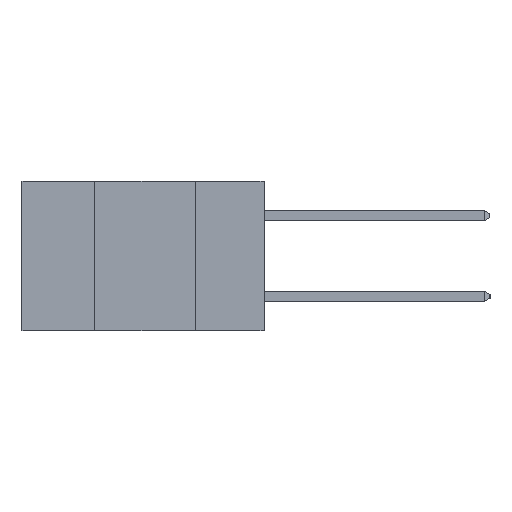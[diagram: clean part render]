
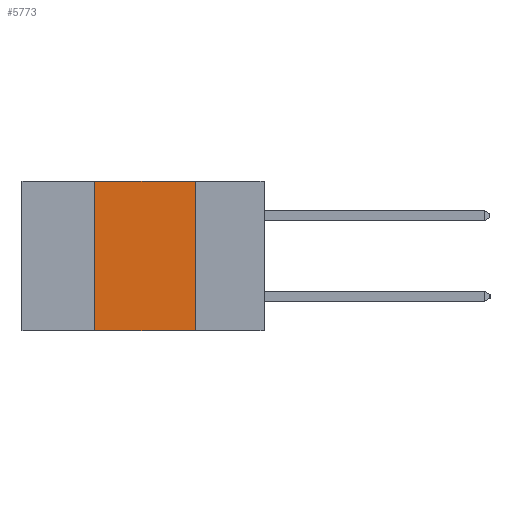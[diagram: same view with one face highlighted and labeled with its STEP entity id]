
A CAD part, left-side view. The second image highlights one B-rep face of the part: STEP entity #5773.
In plain terms, the highlighted planar face has unit normal (-1, 0, 0).
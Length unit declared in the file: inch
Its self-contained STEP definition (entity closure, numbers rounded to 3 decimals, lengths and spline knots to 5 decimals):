
#459 = LINE ( 'NONE', #12350, #6784 ) ;
#1414 = DIRECTION ( 'NONE',  ( 0., -1., 0. ) ) ;
#1646 = ORIENTED_EDGE ( 'NONE', *, *, #6915, .F. ) ;
#1975 = DIRECTION ( 'NONE',  ( 0., 0., -1. ) ) ;
#2228 = DIRECTION ( 'NONE',  ( 0., -1., 0. ) ) ;
#2509 = ORIENTED_EDGE ( 'NONE', *, *, #5936, .T. ) ;
#3166 = PLANE ( 'NONE',  #3678 ) ;
#3678 = AXIS2_PLACEMENT_3D ( 'NONE', #12093, #4414, #13407 ) ;
#3845 = VERTEX_POINT ( 'NONE', #4619 ) ;
#4414 = DIRECTION ( 'NONE',  ( 1., 0., 0. ) ) ;
#4619 = CARTESIAN_POINT ( 'NONE',  ( 0., 0.17, -0.37 ) ) ;
#5125 = EDGE_CURVE ( 'NONE', #7775, #3845, #15491, .T. ) ;
#5773 = ADVANCED_FACE ( 'NONE', ( #9218 ), #3166, .F. ) ;
#5936 = EDGE_CURVE ( 'NONE', #16485, #3845, #459, .T. ) ;
#6454 = CARTESIAN_POINT ( 'NONE',  ( 0., 0.6, 0. ) ) ;
#6779 = CARTESIAN_POINT ( 'NONE',  ( 0., 0.42, -0.37 ) ) ;
#6784 = VECTOR ( 'NONE', #2228, 39.37008 ) ;
#6915 = EDGE_CURVE ( 'NONE', #16485, #11255, #11955, .T. ) ;
#7523 = CARTESIAN_POINT ( 'NONE',  ( 0., 0.42, 0. ) ) ;
#7775 = VERTEX_POINT ( 'NONE', #9191 ) ;
#8298 = CARTESIAN_POINT ( 'NONE',  ( 0., 0.17, -0.37 ) ) ;
#8554 = VECTOR ( 'NONE', #12859, 39.37008 ) ;
#8820 = LINE ( 'NONE', #6454, #15690 ) ;
#9191 = CARTESIAN_POINT ( 'NONE',  ( 0., 0.17, 0. ) ) ;
#9218 = FACE_OUTER_BOUND ( 'NONE', #13892, .T. ) ;
#10274 = CARTESIAN_POINT ( 'NONE',  ( 0., 0.42, -0.37 ) ) ;
#10815 = ORIENTED_EDGE ( 'NONE', *, *, #5125, .F. ) ;
#11255 = VERTEX_POINT ( 'NONE', #7523 ) ;
#11281 = ORIENTED_EDGE ( 'NONE', *, *, #12345, .F. ) ;
#11627 = VECTOR ( 'NONE', #1975, 39.37008 ) ;
#11955 = LINE ( 'NONE', #10274, #8554 ) ;
#12093 = CARTESIAN_POINT ( 'NONE',  ( 0., 0.6, 0. ) ) ;
#12345 = EDGE_CURVE ( 'NONE', #11255, #7775, #8820, .T. ) ;
#12350 = CARTESIAN_POINT ( 'NONE',  ( 0., 0.6, -0.37 ) ) ;
#12859 = DIRECTION ( 'NONE',  ( 0., 0., 1. ) ) ;
#13407 = DIRECTION ( 'NONE',  ( 0., 0., -1. ) ) ;
#13892 = EDGE_LOOP ( 'NONE', ( #10815, #11281, #1646, #2509 ) ) ;
#15491 = LINE ( 'NONE', #8298, #11627 ) ;
#15690 = VECTOR ( 'NONE', #1414, 39.37008 ) ;
#16485 = VERTEX_POINT ( 'NONE', #6779 ) ;
